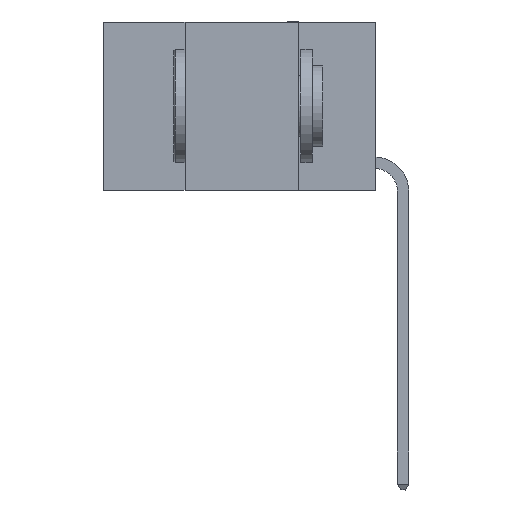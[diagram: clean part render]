
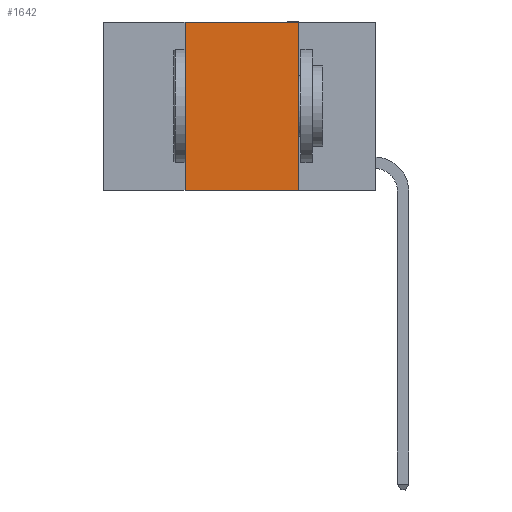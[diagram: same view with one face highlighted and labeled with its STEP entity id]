
A CAD part, left-side view. The second image highlights one B-rep face of the part: STEP entity #1642.
In plain terms, the highlighted planar face has unit normal (-1, 0, 0).
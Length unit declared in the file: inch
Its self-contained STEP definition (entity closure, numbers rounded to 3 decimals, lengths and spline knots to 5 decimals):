
#314 = ORIENTED_EDGE ( 'NONE', *, *, #977, .T. ) ;
#501 = DIRECTION ( 'NONE',  ( 0., 0., -1. ) ) ;
#506 = VECTOR ( 'NONE', #7840, 39.37008 ) ;
#972 = DIRECTION ( 'NONE',  ( 0., -1., 0. ) ) ;
#977 = EDGE_CURVE ( 'NONE', #11905, #12820, #8241, .T. ) ;
#1616 = LINE ( 'NONE', #7766, #506 ) ;
#1631 = EDGE_LOOP ( 'NONE', ( #2391, #20046, #17634, #314 ) ) ;
#1642 = ADVANCED_FACE ( 'NONE', ( #8483 ), #15944, .F. ) ;
#2391 = ORIENTED_EDGE ( 'NONE', *, *, #7269, .F. ) ;
#3232 = AXIS2_PLACEMENT_3D ( 'NONE', #22007, #17056, #501 ) ;
#3300 = CARTESIAN_POINT ( 'NONE',  ( 0., 0.17, 0. ) ) ;
#3589 = VECTOR ( 'NONE', #21230, 39.37008 ) ;
#4510 = EDGE_CURVE ( 'NONE', #11905, #19027, #1616, .T. ) ;
#5602 = VECTOR ( 'NONE', #22489, 39.37008 ) ;
#6138 = LINE ( 'NONE', #21848, #19475 ) ;
#7269 = EDGE_CURVE ( 'NONE', #21108, #12820, #10219, .T. ) ;
#7276 = CARTESIAN_POINT ( 'NONE',  ( 0., 0.42, 0. ) ) ;
#7766 = CARTESIAN_POINT ( 'NONE',  ( 0., 0.42, 0. ) ) ;
#7840 = DIRECTION ( 'NONE',  ( 0., 0., 1. ) ) ;
#8241 = LINE ( 'NONE', #19487, #3589 ) ;
#8483 = FACE_OUTER_BOUND ( 'NONE', #1631, .T. ) ;
#10219 = LINE ( 'NONE', #3300, #5602 ) ;
#10607 = CARTESIAN_POINT ( 'NONE',  ( 0., 0.17, -0.37 ) ) ;
#11905 = VERTEX_POINT ( 'NONE', #16351 ) ;
#12820 = VERTEX_POINT ( 'NONE', #10607 ) ;
#13326 = CARTESIAN_POINT ( 'NONE',  ( 0., 0.17, 0. ) ) ;
#15944 = PLANE ( 'NONE',  #3232 ) ;
#16351 = CARTESIAN_POINT ( 'NONE',  ( 0., 0.42, -0.37 ) ) ;
#17056 = DIRECTION ( 'NONE',  ( 1., 0., 0. ) ) ;
#17634 = ORIENTED_EDGE ( 'NONE', *, *, #4510, .F. ) ;
#19027 = VERTEX_POINT ( 'NONE', #7276 ) ;
#19475 = VECTOR ( 'NONE', #972, 39.37008 ) ;
#19487 = CARTESIAN_POINT ( 'NONE',  ( 0., 0.6, -0.37 ) ) ;
#20046 = ORIENTED_EDGE ( 'NONE', *, *, #20337, .F. ) ;
#20337 = EDGE_CURVE ( 'NONE', #19027, #21108, #6138, .T. ) ;
#21108 = VERTEX_POINT ( 'NONE', #13326 ) ;
#21230 = DIRECTION ( 'NONE',  ( 0., -1., 0. ) ) ;
#21848 = CARTESIAN_POINT ( 'NONE',  ( 0., 0.6, 0. ) ) ;
#22007 = CARTESIAN_POINT ( 'NONE',  ( 0., 0.6, 0. ) ) ;
#22489 = DIRECTION ( 'NONE',  ( 0., 0., -1. ) ) ;
